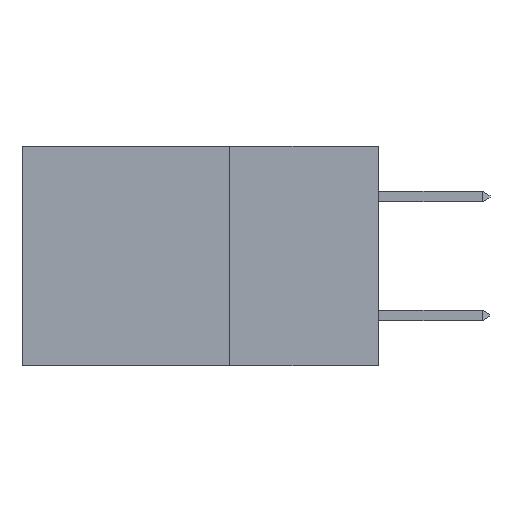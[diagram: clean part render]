
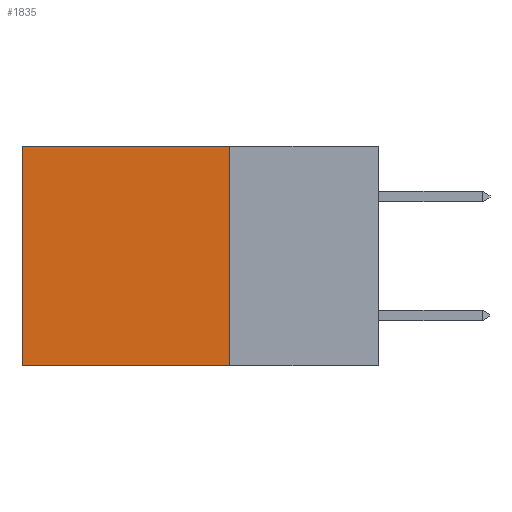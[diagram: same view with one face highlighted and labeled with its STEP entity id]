
A CAD part, left-side view. The second image highlights one B-rep face of the part: STEP entity #1835.
In plain terms, the highlighted planar face has unit normal (-1, 0, 0).
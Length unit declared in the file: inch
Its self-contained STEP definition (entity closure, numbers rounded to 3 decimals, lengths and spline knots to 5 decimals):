
#206 = CARTESIAN_POINT ( 'NONE',  ( 0.298, 0.25, 0. ) ) ;
#456 = VECTOR ( 'NONE', #19461, 39.37008 ) ;
#1536 = LINE ( 'NONE', #5173, #456 ) ;
#1775 = VERTEX_POINT ( 'NONE', #6306 ) ;
#1835 = ADVANCED_FACE ( 'NONE', ( #15279 ), #22438, .F. ) ;
#2780 = DIRECTION ( 'NONE',  ( 0., 0., -1. ) ) ;
#2809 = DIRECTION ( 'NONE',  ( 1., 0., 0. ) ) ;
#3010 = LINE ( 'NONE', #206, #11366 ) ;
#3900 = CARTESIAN_POINT ( 'NONE',  ( 0.298, 0.25, -0.37 ) ) ;
#4010 = CARTESIAN_POINT ( 'NONE',  ( 0.298, 0.25, -0.37 ) ) ;
#4381 = VERTEX_POINT ( 'NONE', #4010 ) ;
#4981 = VECTOR ( 'NONE', #2780, 39.37008 ) ;
#5173 = CARTESIAN_POINT ( 'NONE',  ( 0.298, 0.25, 0. ) ) ;
#5603 = DIRECTION ( 'NONE',  ( 0., 0., -1. ) ) ;
#6306 = CARTESIAN_POINT ( 'NONE',  ( 0.298, 0.6, 0. ) ) ;
#6415 = VERTEX_POINT ( 'NONE', #22568 ) ;
#7019 = AXIS2_PLACEMENT_3D ( 'NONE', #8216, #2809, #5603 ) ;
#8012 = VECTOR ( 'NONE', #18195, 39.37008 ) ;
#8216 = CARTESIAN_POINT ( 'NONE',  ( 0.298, 0.25, 0. ) ) ;
#8270 = ORIENTED_EDGE ( 'NONE', *, *, #9606, .T. ) ;
#9025 = DIRECTION ( 'NONE',  ( 0., 1., 0. ) ) ;
#9162 = LINE ( 'NONE', #13443, #4981 ) ;
#9606 = EDGE_CURVE ( 'NONE', #21992, #1775, #3010, .T. ) ;
#9910 = EDGE_CURVE ( 'NONE', #1775, #6415, #9162, .T. ) ;
#10367 = ORIENTED_EDGE ( 'NONE', *, *, #12913, .F. ) ;
#10965 = ORIENTED_EDGE ( 'NONE', *, *, #9910, .T. ) ;
#11047 = EDGE_CURVE ( 'NONE', #4381, #6415, #17557, .T. ) ;
#11366 = VECTOR ( 'NONE', #9025, 39.37008 ) ;
#12913 = EDGE_CURVE ( 'NONE', #21992, #4381, #1536, .T. ) ;
#13443 = CARTESIAN_POINT ( 'NONE',  ( 0.298, 0.6, 0. ) ) ;
#14384 = ORIENTED_EDGE ( 'NONE', *, *, #11047, .F. ) ;
#15279 = FACE_OUTER_BOUND ( 'NONE', #20963, .T. ) ;
#17557 = LINE ( 'NONE', #3900, #8012 ) ;
#18195 = DIRECTION ( 'NONE',  ( 0., 1., 0. ) ) ;
#19461 = DIRECTION ( 'NONE',  ( 0., 0., -1. ) ) ;
#20963 = EDGE_LOOP ( 'NONE', ( #10965, #14384, #10367, #8270 ) ) ;
#21022 = CARTESIAN_POINT ( 'NONE',  ( 0.298, 0.25, 0. ) ) ;
#21992 = VERTEX_POINT ( 'NONE', #21022 ) ;
#22438 = PLANE ( 'NONE',  #7019 ) ;
#22568 = CARTESIAN_POINT ( 'NONE',  ( 0.298, 0.6, -0.37 ) ) ;
